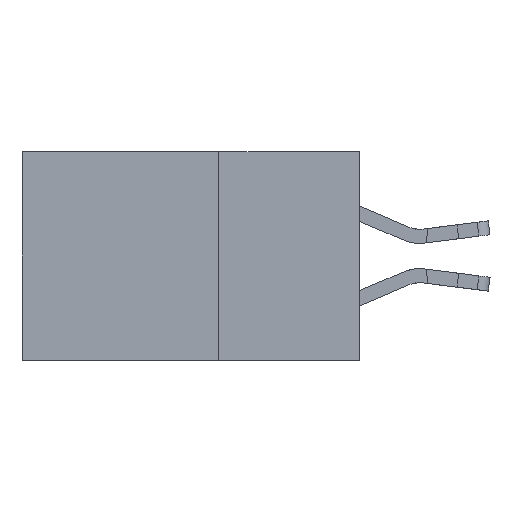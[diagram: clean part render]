
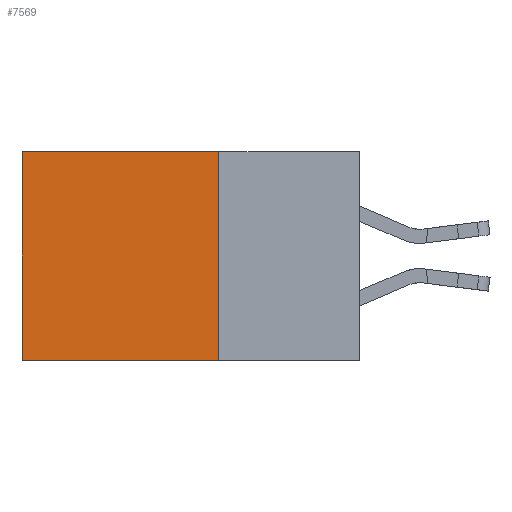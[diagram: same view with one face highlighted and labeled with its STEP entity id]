
A CAD part, left-side view. The second image highlights one B-rep face of the part: STEP entity #7569.
In plain terms, the highlighted planar face has unit normal (-1, 0, 0).
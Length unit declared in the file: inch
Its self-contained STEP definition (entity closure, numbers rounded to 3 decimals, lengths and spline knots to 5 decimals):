
#199 = LINE ( 'NONE', #13664, #21176 ) ;
#371 = EDGE_CURVE ( 'NONE', #20229, #2056, #21161, .T. ) ;
#581 = ORIENTED_EDGE ( 'NONE', *, *, #371, .T. ) ;
#1002 = DIRECTION ( 'NONE',  ( 0., 1., 0. ) ) ;
#1484 = CARTESIAN_POINT ( 'NONE',  ( 0.2875, 0.25, -0.37 ) ) ;
#2056 = VERTEX_POINT ( 'NONE', #15640 ) ;
#2712 = VECTOR ( 'NONE', #3657, 39.37008 ) ;
#2755 = DIRECTION ( 'NONE',  ( 0., 0., -1. ) ) ;
#3657 = DIRECTION ( 'NONE',  ( 0., 1., 0. ) ) ;
#5582 = DIRECTION ( 'NONE',  ( 0., 0., -1. ) ) ;
#6420 = CARTESIAN_POINT ( 'NONE',  ( 0.2875, 0.25, 0. ) ) ;
#6457 = VERTEX_POINT ( 'NONE', #6420 ) ;
#7569 = ADVANCED_FACE ( 'NONE', ( #9444 ), #19773, .F. ) ;
#9021 = CARTESIAN_POINT ( 'NONE',  ( 0.2875, 0.25, 0. ) ) ;
#9444 = FACE_OUTER_BOUND ( 'NONE', #12055, .T. ) ;
#10842 = DIRECTION ( 'NONE',  ( 1., 0., 0. ) ) ;
#12055 = EDGE_LOOP ( 'NONE', ( #581, #13988, #15281, #20057 ) ) ;
#12799 = VECTOR ( 'NONE', #1002, 39.37008 ) ;
#12881 = VERTEX_POINT ( 'NONE', #1484 ) ;
#12962 = LINE ( 'NONE', #14591, #2712 ) ;
#13343 = EDGE_CURVE ( 'NONE', #6457, #12881, #199, .T. ) ;
#13664 = CARTESIAN_POINT ( 'NONE',  ( 0.2875, 0.25, 0. ) ) ;
#13988 = ORIENTED_EDGE ( 'NONE', *, *, #18989, .F. ) ;
#14591 = CARTESIAN_POINT ( 'NONE',  ( 0.2875, 0.25, 0. ) ) ;
#15281 = ORIENTED_EDGE ( 'NONE', *, *, #13343, .F. ) ;
#15361 = CARTESIAN_POINT ( 'NONE',  ( 0.2875, 0.6, 0. ) ) ;
#15640 = CARTESIAN_POINT ( 'NONE',  ( 0.2875, 0.6, -0.37 ) ) ;
#15901 = VECTOR ( 'NONE', #5582, 39.37008 ) ;
#18989 = EDGE_CURVE ( 'NONE', #12881, #2056, #21760, .T. ) ;
#19387 = AXIS2_PLACEMENT_3D ( 'NONE', #9021, #10842, #23383 ) ;
#19773 = PLANE ( 'NONE',  #19387 ) ;
#20057 = ORIENTED_EDGE ( 'NONE', *, *, #22062, .T. ) ;
#20164 = CARTESIAN_POINT ( 'NONE',  ( 0.2875, 0.6, 0. ) ) ;
#20229 = VERTEX_POINT ( 'NONE', #15361 ) ;
#21161 = LINE ( 'NONE', #20164, #15901 ) ;
#21176 = VECTOR ( 'NONE', #2755, 39.37008 ) ;
#21760 = LINE ( 'NONE', #22653, #12799 ) ;
#22062 = EDGE_CURVE ( 'NONE', #6457, #20229, #12962, .T. ) ;
#22653 = CARTESIAN_POINT ( 'NONE',  ( 0.2875, 0.25, -0.37 ) ) ;
#23383 = DIRECTION ( 'NONE',  ( 0., 0., -1. ) ) ;
